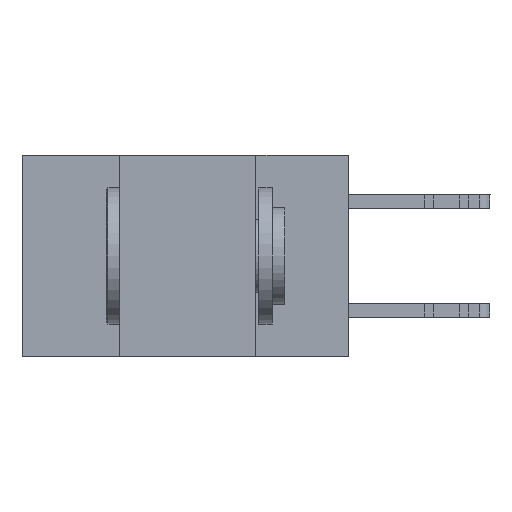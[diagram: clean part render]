
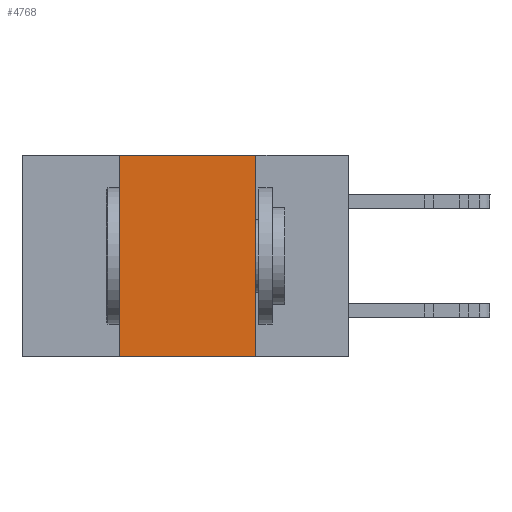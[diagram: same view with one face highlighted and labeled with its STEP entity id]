
A CAD part, left-side view. The second image highlights one B-rep face of the part: STEP entity #4768.
In plain terms, the highlighted planar face has unit normal (-1, 0, 0).
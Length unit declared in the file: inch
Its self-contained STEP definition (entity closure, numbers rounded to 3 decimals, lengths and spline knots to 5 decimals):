
#138 = CARTESIAN_POINT ( 'NONE',  ( 0., 0.42, -0.37 ) ) ;
#905 = CARTESIAN_POINT ( 'NONE',  ( 0., 0.17, -0.37 ) ) ;
#1603 = VECTOR ( 'NONE', #23867, 39.37008 ) ;
#2313 = DIRECTION ( 'NONE',  ( 0., -1., 0. ) ) ;
#2711 = CARTESIAN_POINT ( 'NONE',  ( 0., 0.17, 0. ) ) ;
#4094 = DIRECTION ( 'NONE',  ( 0., 0., -1. ) ) ;
#4768 = ADVANCED_FACE ( 'NONE', ( #11061 ), #15014, .F. ) ;
#4789 = LINE ( 'NONE', #24320, #10110 ) ;
#5527 = LINE ( 'NONE', #12351, #1603 ) ;
#5910 = LINE ( 'NONE', #25720, #16802 ) ;
#6438 = DIRECTION ( 'NONE',  ( 0., 0., 1. ) ) ;
#6869 = ORIENTED_EDGE ( 'NONE', *, *, #18833, .F. ) ;
#7876 = EDGE_CURVE ( 'NONE', #9590, #16589, #5910, .T. ) ;
#8341 = CARTESIAN_POINT ( 'NONE',  ( 0., 0.42, 0. ) ) ;
#9590 = VERTEX_POINT ( 'NONE', #2711 ) ;
#10110 = VECTOR ( 'NONE', #2313, 39.37008 ) ;
#10349 = EDGE_CURVE ( 'NONE', #18610, #9590, #4789, .T. ) ;
#11061 = FACE_OUTER_BOUND ( 'NONE', #28138, .T. ) ;
#12351 = CARTESIAN_POINT ( 'NONE',  ( 0., 0.6, -0.37 ) ) ;
#12830 = VECTOR ( 'NONE', #6438, 39.37008 ) ;
#15014 = PLANE ( 'NONE',  #25605 ) ;
#16589 = VERTEX_POINT ( 'NONE', #905 ) ;
#16802 = VECTOR ( 'NONE', #26009, 39.37008 ) ;
#17174 = EDGE_CURVE ( 'NONE', #18138, #16589, #5527, .T. ) ;
#17352 = CARTESIAN_POINT ( 'NONE',  ( 0., 0.6, 0. ) ) ;
#17364 = LINE ( 'NONE', #8341, #12830 ) ;
#18138 = VERTEX_POINT ( 'NONE', #138 ) ;
#18610 = VERTEX_POINT ( 'NONE', #24817 ) ;
#18833 = EDGE_CURVE ( 'NONE', #18138, #18610, #17364, .T. ) ;
#19260 = ORIENTED_EDGE ( 'NONE', *, *, #10349, .F. ) ;
#19824 = DIRECTION ( 'NONE',  ( 1., 0., 0. ) ) ;
#22769 = ORIENTED_EDGE ( 'NONE', *, *, #17174, .T. ) ;
#23438 = ORIENTED_EDGE ( 'NONE', *, *, #7876, .F. ) ;
#23867 = DIRECTION ( 'NONE',  ( 0., -1., 0. ) ) ;
#24320 = CARTESIAN_POINT ( 'NONE',  ( 0., 0.6, 0. ) ) ;
#24817 = CARTESIAN_POINT ( 'NONE',  ( 0., 0.42, 0. ) ) ;
#25605 = AXIS2_PLACEMENT_3D ( 'NONE', #17352, #19824, #4094 ) ;
#25720 = CARTESIAN_POINT ( 'NONE',  ( 0., 0.17, 0. ) ) ;
#26009 = DIRECTION ( 'NONE',  ( 0., 0., -1. ) ) ;
#28138 = EDGE_LOOP ( 'NONE', ( #23438, #19260, #6869, #22769 ) ) ;
